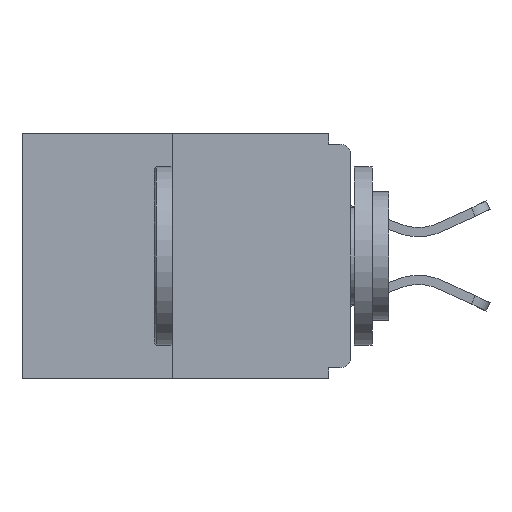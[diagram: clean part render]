
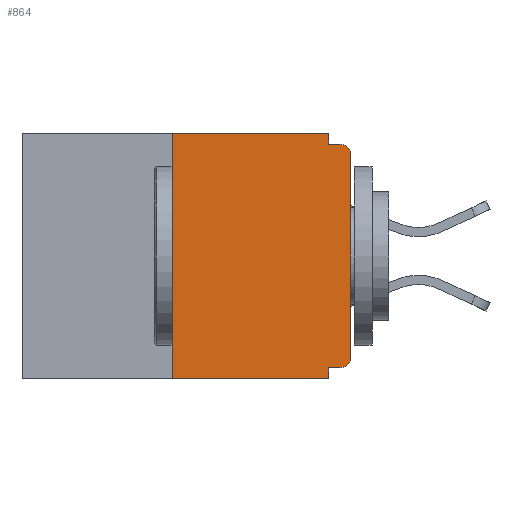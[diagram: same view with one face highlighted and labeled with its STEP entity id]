
A CAD part, left-side view. The second image highlights one B-rep face of the part: STEP entity #864.
In plain terms, the highlighted planar face has unit normal (-1, 0, 0).
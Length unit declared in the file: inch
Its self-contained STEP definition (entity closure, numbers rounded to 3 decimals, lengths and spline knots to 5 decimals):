
#81 = EDGE_CURVE ( 'NONE', #25443, #23380, #13609, .T. ) ;
#851 = ORIENTED_EDGE ( 'NONE', *, *, #81, .T. ) ;
#864 = ADVANCED_FACE ( 'NONE', ( #6424 ), #24168, .F. ) ;
#1211 = EDGE_CURVE ( 'NONE', #23380, #15401, #17037, .T. ) ;
#1235 = VECTOR ( 'NONE', #9007, 39.37008 ) ;
#1831 = EDGE_CURVE ( 'NONE', #21063, #17802, #4645, .T. ) ;
#2292 = LINE ( 'NONE', #9716, #25024 ) ;
#2538 = EDGE_LOOP ( 'NONE', ( #11996, #18368, #7715, #14408, #19958, #2740, #851, #9964, #17753, #12566 ) ) ;
#2712 = DIRECTION ( 'NONE',  ( 0., 0., -1. ) ) ;
#2740 = ORIENTED_EDGE ( 'NONE', *, *, #25303, .T. ) ;
#2985 = VECTOR ( 'NONE', #24720, 39.37008 ) ;
#3418 = VECTOR ( 'NONE', #6541, 39.37008 ) ;
#4165 = CIRCLE ( 'NONE', #19868, 0.015 ) ;
#4645 = LINE ( 'NONE', #24539, #27384 ) ;
#4784 = LINE ( 'NONE', #15645, #3418 ) ;
#4795 = VERTEX_POINT ( 'NONE', #15389 ) ;
#5287 = CARTESIAN_POINT ( 'NONE',  ( 0., 0.46, 0. ) ) ;
#5581 = DIRECTION ( 'NONE',  ( 0., -1., 0. ) ) ;
#5802 = VERTEX_POINT ( 'NONE', #17361 ) ;
#5970 = DIRECTION ( 'NONE',  ( -1., 0., 0. ) ) ;
#6424 = FACE_OUTER_BOUND ( 'NONE', #2538, .T. ) ;
#6541 = DIRECTION ( 'NONE',  ( 0., 1., 0. ) ) ;
#6764 = DIRECTION ( 'NONE',  ( 1., 0., 0. ) ) ;
#7188 = LINE ( 'NONE', #27561, #18203 ) ;
#7715 = ORIENTED_EDGE ( 'NONE', *, *, #10560, .T. ) ;
#7771 = VECTOR ( 'NONE', #15270, 39.37008 ) ;
#7816 = DIRECTION ( 'NONE',  ( 0., 0., 1. ) ) ;
#7978 = CARTESIAN_POINT ( 'NONE',  ( 0., 0.015, -0.328 ) ) ;
#8901 = CARTESIAN_POINT ( 'NONE',  ( 0., 0.015, -0.015 ) ) ;
#9007 = DIRECTION ( 'NONE',  ( 0., 0., -1. ) ) ;
#9716 = CARTESIAN_POINT ( 'NONE',  ( 0., 0.46, -0.343 ) ) ;
#9964 = ORIENTED_EDGE ( 'NONE', *, *, #1211, .T. ) ;
#10560 = EDGE_CURVE ( 'NONE', #4795, #21556, #2292, .T. ) ;
#10648 = VERTEX_POINT ( 'NONE', #16894 ) ;
#11850 = CARTESIAN_POINT ( 'NONE',  ( 0., 0., -0.313 ) ) ;
#11996 = ORIENTED_EDGE ( 'NONE', *, *, #14023, .F. ) ;
#12566 = ORIENTED_EDGE ( 'NONE', *, *, #1831, .F. ) ;
#12600 = LINE ( 'NONE', #5287, #2985 ) ;
#13298 = DIRECTION ( 'NONE',  ( 0., 0., -1. ) ) ;
#13380 = DIRECTION ( 'NONE',  ( 0., 0., -1. ) ) ;
#13609 = LINE ( 'NONE', #15449, #7771 ) ;
#13785 = VERTEX_POINT ( 'NONE', #7978 ) ;
#14018 = DIRECTION ( 'NONE',  ( 0., -1., 0. ) ) ;
#14023 = EDGE_CURVE ( 'NONE', #5802, #21063, #12600, .T. ) ;
#14408 = ORIENTED_EDGE ( 'NONE', *, *, #22537, .F. ) ;
#15270 = DIRECTION ( 'NONE',  ( 0., 0., 1. ) ) ;
#15389 = CARTESIAN_POINT ( 'NONE',  ( 0., 0.25, -0.343 ) ) ;
#15401 = VERTEX_POINT ( 'NONE', #8901 ) ;
#15449 = CARTESIAN_POINT ( 'NONE',  ( 0., 0., 0. ) ) ;
#15645 = CARTESIAN_POINT ( 'NONE',  ( 0., 0., -0.328 ) ) ;
#15665 = LINE ( 'NONE', #22791, #21172 ) ;
#15849 = DIRECTION ( 'NONE',  ( -1., 0., 0. ) ) ;
#16894 = CARTESIAN_POINT ( 'NONE',  ( 0., 0.031, -0.328 ) ) ;
#17037 = CIRCLE ( 'NONE', #27595, 0.015 ) ;
#17083 = CARTESIAN_POINT ( 'NONE',  ( 0., 0.015, -0.03 ) ) ;
#17201 = AXIS2_PLACEMENT_3D ( 'NONE', #17515, #6764, #13298 ) ;
#17361 = CARTESIAN_POINT ( 'NONE',  ( 0., 0.25, 0. ) ) ;
#17515 = CARTESIAN_POINT ( 'NONE',  ( 0., 0.46, 0. ) ) ;
#17753 = ORIENTED_EDGE ( 'NONE', *, *, #22314, .F. ) ;
#17802 = VERTEX_POINT ( 'NONE', #26302 ) ;
#17991 = CARTESIAN_POINT ( 'NONE',  ( 0., 0.015, -0.313 ) ) ;
#18203 = VECTOR ( 'NONE', #7816, 39.37008 ) ;
#18368 = ORIENTED_EDGE ( 'NONE', *, *, #20702, .F. ) ;
#19868 = AXIS2_PLACEMENT_3D ( 'NONE', #17991, #15849, #13380 ) ;
#19958 = ORIENTED_EDGE ( 'NONE', *, *, #20888, .F. ) ;
#20702 = EDGE_CURVE ( 'NONE', #4795, #5802, #7188, .T. ) ;
#20888 = EDGE_CURVE ( 'NONE', #13785, #10648, #4784, .T. ) ;
#21063 = VERTEX_POINT ( 'NONE', #24639 ) ;
#21172 = VECTOR ( 'NONE', #14018, 39.37008 ) ;
#21556 = VERTEX_POINT ( 'NONE', #22276 ) ;
#22276 = CARTESIAN_POINT ( 'NONE',  ( 0., 0.031, -0.343 ) ) ;
#22314 = EDGE_CURVE ( 'NONE', #17802, #15401, #15665, .T. ) ;
#22537 = EDGE_CURVE ( 'NONE', #10648, #21556, #23595, .T. ) ;
#22791 = CARTESIAN_POINT ( 'NONE',  ( 0., 0., -0.015 ) ) ;
#23380 = VERTEX_POINT ( 'NONE', #24541 ) ;
#23595 = LINE ( 'NONE', #24098, #1235 ) ;
#24098 = CARTESIAN_POINT ( 'NONE',  ( 0., 0.031, -0.343 ) ) ;
#24168 = PLANE ( 'NONE',  #17201 ) ;
#24539 = CARTESIAN_POINT ( 'NONE',  ( 0., 0.031, 0. ) ) ;
#24541 = CARTESIAN_POINT ( 'NONE',  ( 0., 0., -0.03 ) ) ;
#24639 = CARTESIAN_POINT ( 'NONE',  ( 0., 0.031, 0. ) ) ;
#24720 = DIRECTION ( 'NONE',  ( 0., -1., 0. ) ) ;
#25024 = VECTOR ( 'NONE', #5581, 39.37008 ) ;
#25303 = EDGE_CURVE ( 'NONE', #13785, #25443, #4165, .T. ) ;
#25443 = VERTEX_POINT ( 'NONE', #11850 ) ;
#25622 = DIRECTION ( 'NONE',  ( 0., 0., -1. ) ) ;
#26302 = CARTESIAN_POINT ( 'NONE',  ( 0., 0.031, -0.015 ) ) ;
#27384 = VECTOR ( 'NONE', #2712, 39.37008 ) ;
#27561 = CARTESIAN_POINT ( 'NONE',  ( 0., 0.25, 0. ) ) ;
#27595 = AXIS2_PLACEMENT_3D ( 'NONE', #17083, #5970, #25622 ) ;
